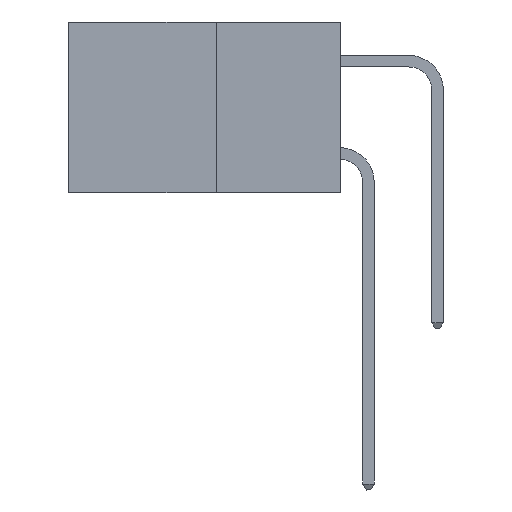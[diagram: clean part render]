
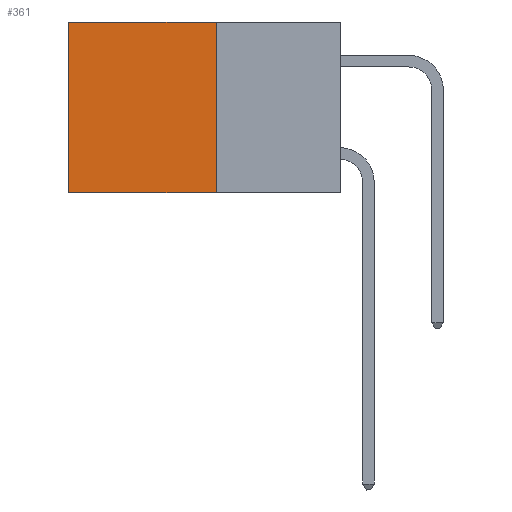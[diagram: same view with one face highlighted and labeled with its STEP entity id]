
A CAD part, left-side view. The second image highlights one B-rep face of the part: STEP entity #361.
In plain terms, the highlighted planar face has unit normal (-1, 0, 0).
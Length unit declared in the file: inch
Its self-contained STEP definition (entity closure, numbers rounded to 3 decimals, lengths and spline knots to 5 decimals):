
#361 = ADVANCED_FACE ( 'NONE', ( #3447 ), #22906, .F. ) ;
#814 = DIRECTION ( 'NONE',  ( 0., 0., -1. ) ) ;
#2823 = ORIENTED_EDGE ( 'NONE', *, *, #30115, .T. ) ;
#3212 = VERTEX_POINT ( 'NONE', #30235 ) ;
#3289 = VECTOR ( 'NONE', #17374, 39.37008 ) ;
#3447 = FACE_OUTER_BOUND ( 'NONE', #7111, .T. ) ;
#3684 = AXIS2_PLACEMENT_3D ( 'NONE', #13637, #20707, #16655 ) ;
#3993 = EDGE_CURVE ( 'NONE', #10995, #6307, #18350, .T. ) ;
#4801 = ORIENTED_EDGE ( 'NONE', *, *, #8698, .T. ) ;
#6307 = VERTEX_POINT ( 'NONE', #6971 ) ;
#6971 = CARTESIAN_POINT ( 'NONE',  ( 0.277, 0.27, -0.37 ) ) ;
#7111 = EDGE_LOOP ( 'NONE', ( #4801, #21924, #15546, #2823 ) ) ;
#8698 = EDGE_CURVE ( 'NONE', #3212, #11512, #26569, .T. ) ;
#9965 = CARTESIAN_POINT ( 'NONE',  ( 0.277, 0.27, -0.37 ) ) ;
#10995 = VERTEX_POINT ( 'NONE', #16995 ) ;
#11512 = VERTEX_POINT ( 'NONE', #28644 ) ;
#12239 = CARTESIAN_POINT ( 'NONE',  ( 0.277, 0.27, -0.37 ) ) ;
#12531 = DIRECTION ( 'NONE',  ( 0., 1., 0. ) ) ;
#13630 = VECTOR ( 'NONE', #12531, 39.37008 ) ;
#13637 = CARTESIAN_POINT ( 'NONE',  ( 0.277, 0.27, -0.37 ) ) ;
#15546 = ORIENTED_EDGE ( 'NONE', *, *, #3993, .F. ) ;
#16289 = CARTESIAN_POINT ( 'NONE',  ( 0.277, 0.27, 0. ) ) ;
#16612 = VECTOR ( 'NONE', #18815, 39.37008 ) ;
#16655 = DIRECTION ( 'NONE',  ( 0., 0., -1. ) ) ;
#16995 = CARTESIAN_POINT ( 'NONE',  ( 0.277, 0.27, 0. ) ) ;
#17374 = DIRECTION ( 'NONE',  ( 0., 0., -1. ) ) ;
#18350 = LINE ( 'NONE', #12239, #3289 ) ;
#18563 = CARTESIAN_POINT ( 'NONE',  ( 0.277, 0.59, -0.37 ) ) ;
#18815 = DIRECTION ( 'NONE',  ( 0., 1., 0. ) ) ;
#19203 = VECTOR ( 'NONE', #814, 39.37008 ) ;
#20707 = DIRECTION ( 'NONE',  ( 1., 0., 0. ) ) ;
#21924 = ORIENTED_EDGE ( 'NONE', *, *, #28414, .F. ) ;
#22906 = PLANE ( 'NONE',  #3684 ) ;
#26569 = LINE ( 'NONE', #18563, #19203 ) ;
#26833 = LINE ( 'NONE', #9965, #13630 ) ;
#28414 = EDGE_CURVE ( 'NONE', #6307, #11512, #26833, .T. ) ;
#28644 = CARTESIAN_POINT ( 'NONE',  ( 0.277, 0.59, -0.37 ) ) ;
#29794 = LINE ( 'NONE', #16289, #16612 ) ;
#30115 = EDGE_CURVE ( 'NONE', #10995, #3212, #29794, .T. ) ;
#30235 = CARTESIAN_POINT ( 'NONE',  ( 0.277, 0.59, 0. ) ) ;
